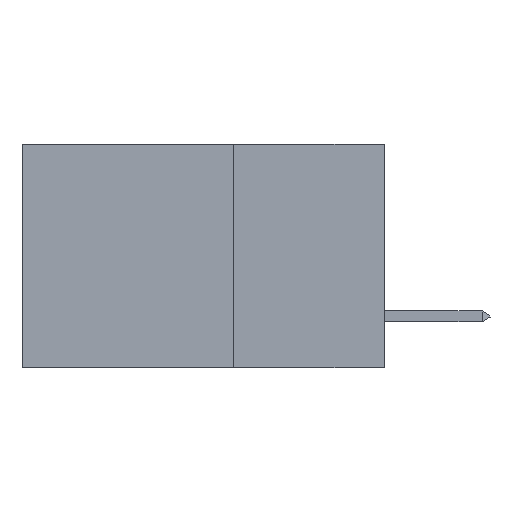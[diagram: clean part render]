
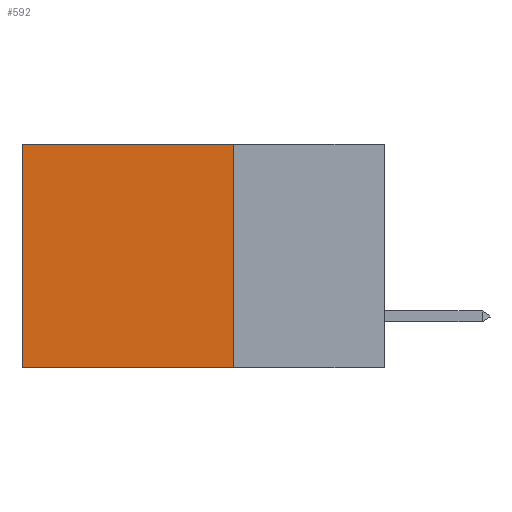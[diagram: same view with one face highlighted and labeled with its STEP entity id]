
A CAD part, left-side view. The second image highlights one B-rep face of the part: STEP entity #592.
In plain terms, the highlighted planar face has unit normal (-1, 0, 0).
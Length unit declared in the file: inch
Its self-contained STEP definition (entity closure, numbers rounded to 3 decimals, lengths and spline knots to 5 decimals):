
#14 = CARTESIAN_POINT ( 'NONE',  ( 0.2875, 0.6, 0. ) ) ;
#298 = AXIS2_PLACEMENT_3D ( 'NONE', #15674, #1195, #5188 ) ;
#592 = ADVANCED_FACE ( 'NONE', ( #15001 ), #7253, .F. ) ;
#1195 = DIRECTION ( 'NONE',  ( 1., 0., 0. ) ) ;
#1791 = DIRECTION ( 'NONE',  ( 0., 1., 0. ) ) ;
#3298 = CARTESIAN_POINT ( 'NONE',  ( 0.2875, 0.25, 0. ) ) ;
#4040 = EDGE_CURVE ( 'NONE', #15484, #6780, #7696, .T. ) ;
#4414 = ORIENTED_EDGE ( 'NONE', *, *, #22161, .F. ) ;
#4479 = DIRECTION ( 'NONE',  ( 0., 1., 0. ) ) ;
#5188 = DIRECTION ( 'NONE',  ( 0., 0., -1. ) ) ;
#6346 = ORIENTED_EDGE ( 'NONE', *, *, #17507, .T. ) ;
#6780 = VERTEX_POINT ( 'NONE', #14 ) ;
#7253 = PLANE ( 'NONE',  #298 ) ;
#7696 = LINE ( 'NONE', #20270, #21596 ) ;
#7779 = CARTESIAN_POINT ( 'NONE',  ( 0.2875, 0.25, -0.37 ) ) ;
#7817 = DIRECTION ( 'NONE',  ( 0., 0., -1. ) ) ;
#8612 = DIRECTION ( 'NONE',  ( 0., 0., -1. ) ) ;
#8876 = EDGE_LOOP ( 'NONE', ( #6346, #4414, #18407, #25381 ) ) ;
#9152 = CARTESIAN_POINT ( 'NONE',  ( 0.2875, 0.25, 0. ) ) ;
#12203 = EDGE_CURVE ( 'NONE', #15484, #24945, #25444, .T. ) ;
#12435 = VECTOR ( 'NONE', #7817, 39.37008 ) ;
#15001 = FACE_OUTER_BOUND ( 'NONE', #8876, .T. ) ;
#15236 = VECTOR ( 'NONE', #4479, 39.37008 ) ;
#15484 = VERTEX_POINT ( 'NONE', #3298 ) ;
#15674 = CARTESIAN_POINT ( 'NONE',  ( 0.2875, 0.25, 0. ) ) ;
#15872 = LINE ( 'NONE', #23073, #15236 ) ;
#16408 = CARTESIAN_POINT ( 'NONE',  ( 0.2875, 0.6, -0.37 ) ) ;
#17507 = EDGE_CURVE ( 'NONE', #6780, #25047, #20201, .T. ) ;
#18407 = ORIENTED_EDGE ( 'NONE', *, *, #12203, .F. ) ;
#20179 = CARTESIAN_POINT ( 'NONE',  ( 0.2875, 0.6, 0. ) ) ;
#20201 = LINE ( 'NONE', #20179, #12435 ) ;
#20270 = CARTESIAN_POINT ( 'NONE',  ( 0.2875, 0.25, 0. ) ) ;
#21596 = VECTOR ( 'NONE', #1791, 39.37008 ) ;
#22161 = EDGE_CURVE ( 'NONE', #24945, #25047, #15872, .T. ) ;
#23073 = CARTESIAN_POINT ( 'NONE',  ( 0.2875, 0.25, -0.37 ) ) ;
#24792 = VECTOR ( 'NONE', #8612, 39.37008 ) ;
#24945 = VERTEX_POINT ( 'NONE', #7779 ) ;
#25047 = VERTEX_POINT ( 'NONE', #16408 ) ;
#25381 = ORIENTED_EDGE ( 'NONE', *, *, #4040, .T. ) ;
#25444 = LINE ( 'NONE', #9152, #24792 ) ;
